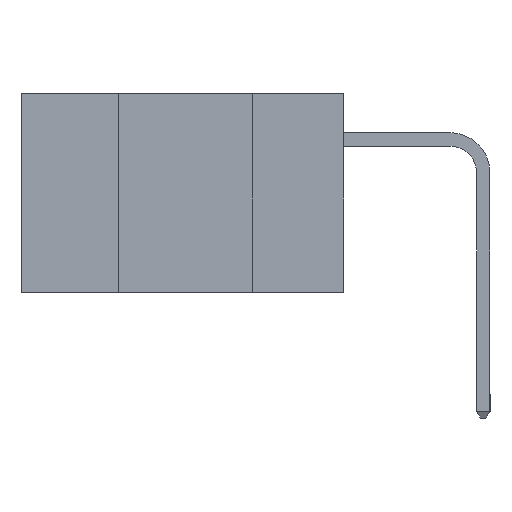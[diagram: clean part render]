
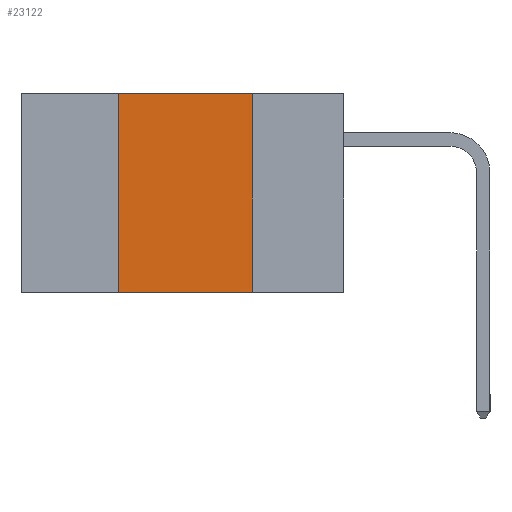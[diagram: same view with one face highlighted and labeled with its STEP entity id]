
A CAD part, left-side view. The second image highlights one B-rep face of the part: STEP entity #23122.
In plain terms, the highlighted planar face has unit normal (-1, 0, 0).
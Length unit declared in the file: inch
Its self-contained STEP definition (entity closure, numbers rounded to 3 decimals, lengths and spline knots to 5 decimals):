
#316 = CARTESIAN_POINT ( 'NONE',  ( 0., 0.17, -0.37 ) ) ;
#549 = VECTOR ( 'NONE', #687, 39.37008 ) ;
#687 = DIRECTION ( 'NONE',  ( 0., 0., -1. ) ) ;
#1741 = VERTEX_POINT ( 'NONE', #13250 ) ;
#3571 = AXIS2_PLACEMENT_3D ( 'NONE', #7621, #20084, #9470 ) ;
#4192 = DIRECTION ( 'NONE',  ( 0., 0., 1. ) ) ;
#4396 = CARTESIAN_POINT ( 'NONE',  ( 0., 0.17, -0.37 ) ) ;
#4402 = CARTESIAN_POINT ( 'NONE',  ( 0., 0.42, -0.37 ) ) ;
#4998 = VECTOR ( 'NONE', #4192, 39.37008 ) ;
#5875 = VERTEX_POINT ( 'NONE', #7422 ) ;
#6382 = VERTEX_POINT ( 'NONE', #316 ) ;
#6472 = ORIENTED_EDGE ( 'NONE', *, *, #16146, .F. ) ;
#6631 = ORIENTED_EDGE ( 'NONE', *, *, #13760, .F. ) ;
#6898 = ORIENTED_EDGE ( 'NONE', *, *, #12563, .F. ) ;
#7069 = ORIENTED_EDGE ( 'NONE', *, *, #11400, .T. ) ;
#7422 = CARTESIAN_POINT ( 'NONE',  ( 0., 0.17, 0. ) ) ;
#7621 = CARTESIAN_POINT ( 'NONE',  ( 0., 0.6, 0. ) ) ;
#8263 = VECTOR ( 'NONE', #17032, 39.37008 ) ;
#9470 = DIRECTION ( 'NONE',  ( 0., 0., -1. ) ) ;
#10905 = LINE ( 'NONE', #4396, #549 ) ;
#11400 = EDGE_CURVE ( 'NONE', #1741, #6382, #22899, .T. ) ;
#12563 = EDGE_CURVE ( 'NONE', #1741, #14444, #14592, .T. ) ;
#13228 = FACE_OUTER_BOUND ( 'NONE', #19617, .T. ) ;
#13250 = CARTESIAN_POINT ( 'NONE',  ( 0., 0.42, -0.37 ) ) ;
#13760 = EDGE_CURVE ( 'NONE', #14444, #5875, #21181, .T. ) ;
#14444 = VERTEX_POINT ( 'NONE', #15778 ) ;
#14592 = LINE ( 'NONE', #4402, #4998 ) ;
#15778 = CARTESIAN_POINT ( 'NONE',  ( 0., 0.42, 0. ) ) ;
#15964 = VECTOR ( 'NONE', #23092, 39.37008 ) ;
#16146 = EDGE_CURVE ( 'NONE', #5875, #6382, #10905, .T. ) ;
#17032 = DIRECTION ( 'NONE',  ( 0., -1., 0. ) ) ;
#17237 = CARTESIAN_POINT ( 'NONE',  ( 0., 0.6, -0.37 ) ) ;
#18297 = PLANE ( 'NONE',  #3571 ) ;
#19617 = EDGE_LOOP ( 'NONE', ( #6472, #6631, #6898, #7069 ) ) ;
#20084 = DIRECTION ( 'NONE',  ( 1., 0., 0. ) ) ;
#21181 = LINE ( 'NONE', #23089, #15964 ) ;
#22899 = LINE ( 'NONE', #17237, #8263 ) ;
#23089 = CARTESIAN_POINT ( 'NONE',  ( 0., 0.6, 0. ) ) ;
#23092 = DIRECTION ( 'NONE',  ( 0., -1., 0. ) ) ;
#23122 = ADVANCED_FACE ( 'NONE', ( #13228 ), #18297, .F. ) ;
